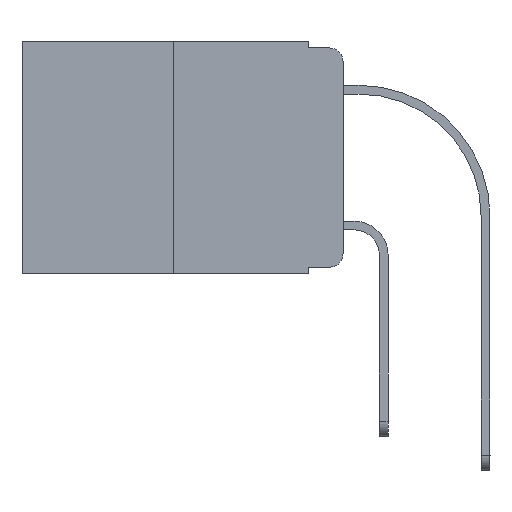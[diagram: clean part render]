
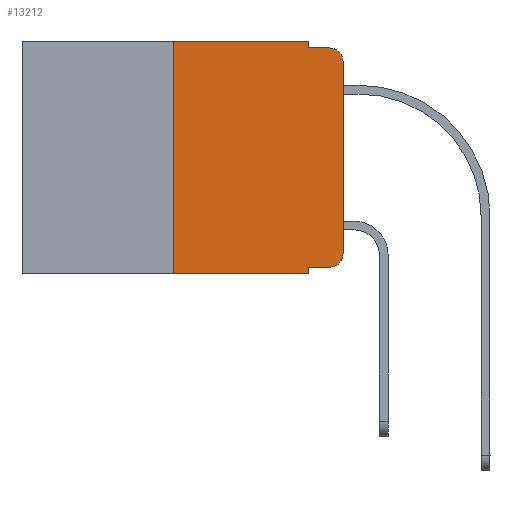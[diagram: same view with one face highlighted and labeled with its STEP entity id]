
A CAD part, left-side view. The second image highlights one B-rep face of the part: STEP entity #13212.
In plain terms, the highlighted planar face has unit normal (-1, 0, 0).
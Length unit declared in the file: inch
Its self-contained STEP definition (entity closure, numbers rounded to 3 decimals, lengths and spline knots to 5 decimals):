
#576 = ORIENTED_EDGE ( 'NONE', *, *, #12837, .F. ) ;
#643 = CIRCLE ( 'NONE', #1438, 0.02 ) ;
#1046 = VECTOR ( 'NONE', #6824, 39.37008 ) ;
#1077 = CARTESIAN_POINT ( 'NONE',  ( 0., 0., 0. ) ) ;
#1208 = CARTESIAN_POINT ( 'NONE',  ( 0., 0.473, 0. ) ) ;
#1438 = AXIS2_PLACEMENT_3D ( 'NONE', #19468, #2360, #9983 ) ;
#1499 = PLANE ( 'NONE',  #8097 ) ;
#2360 = DIRECTION ( 'NONE',  ( -1., 0., 0. ) ) ;
#2495 = DIRECTION ( 'NONE',  ( 0., 0., -1. ) ) ;
#2863 = CARTESIAN_POINT ( 'NONE',  ( 0., 0.051, -0.333 ) ) ;
#3032 = CARTESIAN_POINT ( 'NONE',  ( 0., 0.051, -0.01 ) ) ;
#3164 = CARTESIAN_POINT ( 'NONE',  ( 0., 0.25, -0.343 ) ) ;
#3441 = DIRECTION ( 'NONE',  ( 0., 0., -1. ) ) ;
#3690 = VECTOR ( 'NONE', #15386, 39.37008 ) ;
#4180 = VERTEX_POINT ( 'NONE', #14213 ) ;
#4534 = CARTESIAN_POINT ( 'NONE',  ( 0., 0.25, 0. ) ) ;
#4640 = EDGE_CURVE ( 'NONE', #5220, #12660, #23855, .T. ) ;
#5220 = VERTEX_POINT ( 'NONE', #8794 ) ;
#5364 = VERTEX_POINT ( 'NONE', #3164 ) ;
#6787 = LINE ( 'NONE', #10661, #21694 ) ;
#6824 = DIRECTION ( 'NONE',  ( 0., -1., 0. ) ) ;
#8097 = AXIS2_PLACEMENT_3D ( 'NONE', #18714, #14981, #14478 ) ;
#8120 = VECTOR ( 'NONE', #2495, 39.37008 ) ;
#8498 = LINE ( 'NONE', #2863, #11312 ) ;
#8794 = CARTESIAN_POINT ( 'NONE',  ( 0., 0.051, 0. ) ) ;
#8796 = DIRECTION ( 'NONE',  ( 0., -1., 0. ) ) ;
#8989 = EDGE_CURVE ( 'NONE', #10065, #21958, #643, .T. ) ;
#9058 = EDGE_CURVE ( 'NONE', #19065, #5220, #17817, .T. ) ;
#9400 = VECTOR ( 'NONE', #8796, 39.37008 ) ;
#9559 = DIRECTION ( 'NONE',  ( -1., 0., 0. ) ) ;
#9721 = EDGE_CURVE ( 'NONE', #5364, #20806, #20275, .T. ) ;
#9965 = CIRCLE ( 'NONE', #23919, 0.02 ) ;
#9983 = DIRECTION ( 'NONE',  ( 0., 0., -1. ) ) ;
#10040 = VERTEX_POINT ( 'NONE', #10511 ) ;
#10065 = VERTEX_POINT ( 'NONE', #12496 ) ;
#10362 = DIRECTION ( 'NONE',  ( 0., -1., 0. ) ) ;
#10511 = CARTESIAN_POINT ( 'NONE',  ( 0., 0.051, -0.333 ) ) ;
#10568 = LINE ( 'NONE', #1077, #13720 ) ;
#10661 = CARTESIAN_POINT ( 'NONE',  ( 0., 0.051, 0. ) ) ;
#10831 = ORIENTED_EDGE ( 'NONE', *, *, #11681, .T. ) ;
#10947 = VECTOR ( 'NONE', #22466, 39.37008 ) ;
#11312 = VECTOR ( 'NONE', #10362, 39.37008 ) ;
#11464 = ORIENTED_EDGE ( 'NONE', *, *, #9058, .F. ) ;
#11681 = EDGE_CURVE ( 'NONE', #10040, #10065, #8498, .T. ) ;
#12107 = CARTESIAN_POINT ( 'NONE',  ( 0., 0.051, 0. ) ) ;
#12496 = CARTESIAN_POINT ( 'NONE',  ( 0., 0.02, -0.333 ) ) ;
#12593 = CARTESIAN_POINT ( 'NONE',  ( 0., 0.25, 0. ) ) ;
#12660 = VERTEX_POINT ( 'NONE', #3032 ) ;
#12837 = EDGE_CURVE ( 'NONE', #12660, #13682, #15747, .T. ) ;
#12974 = FACE_OUTER_BOUND ( 'NONE', #15537, .T. ) ;
#12987 = CARTESIAN_POINT ( 'NONE',  ( 0., 0.051, -0.343 ) ) ;
#13212 = ADVANCED_FACE ( 'NONE', ( #12974 ), #1499, .F. ) ;
#13616 = ORIENTED_EDGE ( 'NONE', *, *, #23712, .T. ) ;
#13682 = VERTEX_POINT ( 'NONE', #21820 ) ;
#13720 = VECTOR ( 'NONE', #24044, 39.37008 ) ;
#14213 = CARTESIAN_POINT ( 'NONE',  ( 0., 0., -0.03 ) ) ;
#14478 = DIRECTION ( 'NONE',  ( 0., 0., -1. ) ) ;
#14598 = LINE ( 'NONE', #12593, #10947 ) ;
#14745 = EDGE_CURVE ( 'NONE', #5364, #19065, #14598, .T. ) ;
#14981 = DIRECTION ( 'NONE',  ( 1., 0., 0. ) ) ;
#15386 = DIRECTION ( 'NONE',  ( 0., -1., 0. ) ) ;
#15537 = EDGE_LOOP ( 'NONE', ( #17835, #13616, #576, #21282, #11464, #23818, #19064, #16543, #10831, #22387 ) ) ;
#15747 = LINE ( 'NONE', #19000, #3690 ) ;
#16525 = CARTESIAN_POINT ( 'NONE',  ( 0., 0.473, -0.343 ) ) ;
#16543 = ORIENTED_EDGE ( 'NONE', *, *, #17836, .F. ) ;
#17465 = EDGE_CURVE ( 'NONE', #21958, #4180, #10568, .T. ) ;
#17817 = LINE ( 'NONE', #1208, #1046 ) ;
#17835 = ORIENTED_EDGE ( 'NONE', *, *, #17465, .T. ) ;
#17836 = EDGE_CURVE ( 'NONE', #10040, #20806, #6787, .T. ) ;
#18268 = DIRECTION ( 'NONE',  ( 0., 0., -1. ) ) ;
#18714 = CARTESIAN_POINT ( 'NONE',  ( 0., 0.473, 0. ) ) ;
#19000 = CARTESIAN_POINT ( 'NONE',  ( 0., 0.051, -0.01 ) ) ;
#19064 = ORIENTED_EDGE ( 'NONE', *, *, #9721, .T. ) ;
#19065 = VERTEX_POINT ( 'NONE', #4534 ) ;
#19468 = CARTESIAN_POINT ( 'NONE',  ( 0., 0.02, -0.313 ) ) ;
#20275 = LINE ( 'NONE', #16525, #9400 ) ;
#20666 = CARTESIAN_POINT ( 'NONE',  ( 0., 0.02, -0.03 ) ) ;
#20806 = VERTEX_POINT ( 'NONE', #12987 ) ;
#21282 = ORIENTED_EDGE ( 'NONE', *, *, #4640, .F. ) ;
#21694 = VECTOR ( 'NONE', #18268, 39.37008 ) ;
#21820 = CARTESIAN_POINT ( 'NONE',  ( 0., 0.02, -0.01 ) ) ;
#21958 = VERTEX_POINT ( 'NONE', #22816 ) ;
#22387 = ORIENTED_EDGE ( 'NONE', *, *, #8989, .T. ) ;
#22466 = DIRECTION ( 'NONE',  ( 0., 0., 1. ) ) ;
#22816 = CARTESIAN_POINT ( 'NONE',  ( 0., 0., -0.313 ) ) ;
#23712 = EDGE_CURVE ( 'NONE', #4180, #13682, #9965, .T. ) ;
#23818 = ORIENTED_EDGE ( 'NONE', *, *, #14745, .F. ) ;
#23855 = LINE ( 'NONE', #12107, #8120 ) ;
#23919 = AXIS2_PLACEMENT_3D ( 'NONE', #20666, #9559, #3441 ) ;
#24044 = DIRECTION ( 'NONE',  ( 0., 0., 1. ) ) ;
